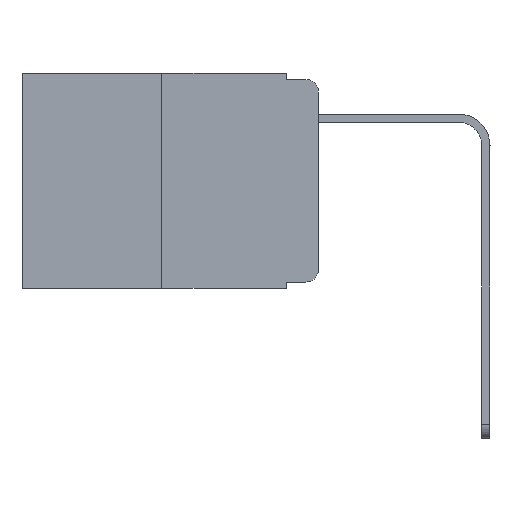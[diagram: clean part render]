
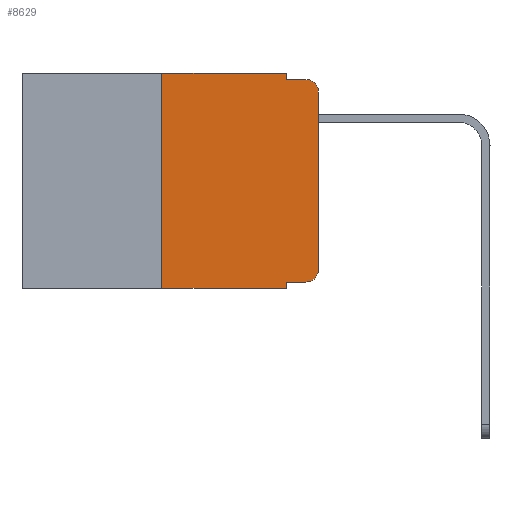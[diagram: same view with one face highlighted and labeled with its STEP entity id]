
A CAD part, left-side view. The second image highlights one B-rep face of the part: STEP entity #8629.
In plain terms, the highlighted planar face has unit normal (-1, 0, 0).
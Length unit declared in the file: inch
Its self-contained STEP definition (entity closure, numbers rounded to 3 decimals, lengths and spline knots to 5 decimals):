
#501 = VERTEX_POINT ( 'NONE', #15920 ) ;
#543 = VECTOR ( 'NONE', #5890, 39.37008 ) ;
#625 = AXIS2_PLACEMENT_3D ( 'NONE', #4485, #13887, #15265 ) ;
#633 = VERTEX_POINT ( 'NONE', #3951 ) ;
#739 = CARTESIAN_POINT ( 'NONE',  ( 0., 0.02, -0.01 ) ) ;
#911 = CARTESIAN_POINT ( 'NONE',  ( 0., 0., -0.03 ) ) ;
#965 = VERTEX_POINT ( 'NONE', #4037 ) ;
#992 = DIRECTION ( 'NONE',  ( 0., -1., 0. ) ) ;
#1010 = DIRECTION ( 'NONE',  ( -1., 0., 0. ) ) ;
#1401 = ORIENTED_EDGE ( 'NONE', *, *, #4761, .F. ) ;
#1824 = VECTOR ( 'NONE', #992, 39.37008 ) ;
#2135 = EDGE_CURVE ( 'NONE', #15957, #16170, #2227, .T. ) ;
#2227 = LINE ( 'NONE', #15925, #16977 ) ;
#2578 = DIRECTION ( 'NONE',  ( 0., 0., -1. ) ) ;
#2835 = DIRECTION ( 'NONE',  ( 0., -1., 0. ) ) ;
#3642 = DIRECTION ( 'NONE',  ( 0., 0., 1. ) ) ;
#3667 = VECTOR ( 'NONE', #15492, 39.37008 ) ;
#3936 = LINE ( 'NONE', #17284, #1824 ) ;
#3951 = CARTESIAN_POINT ( 'NONE',  ( 0., 0.02, -0.333 ) ) ;
#4037 = CARTESIAN_POINT ( 'NONE',  ( 0., 0.051, -0.333 ) ) ;
#4386 = VERTEX_POINT ( 'NONE', #13952 ) ;
#4485 = CARTESIAN_POINT ( 'NONE',  ( 0., 0.473, 0. ) ) ;
#4533 = FACE_OUTER_BOUND ( 'NONE', #6251, .T. ) ;
#4613 = DIRECTION ( 'NONE',  ( 0., 0., 1. ) ) ;
#4761 = EDGE_CURVE ( 'NONE', #4386, #15957, #12010, .T. ) ;
#5108 = LINE ( 'NONE', #12137, #16913 ) ;
#5312 = ORIENTED_EDGE ( 'NONE', *, *, #8524, .F. ) ;
#5323 = CARTESIAN_POINT ( 'NONE',  ( 0., 0.25, 0. ) ) ;
#5349 = ORIENTED_EDGE ( 'NONE', *, *, #17445, .T. ) ;
#5890 = DIRECTION ( 'NONE',  ( 0., 0., -1. ) ) ;
#5933 = VERTEX_POINT ( 'NONE', #739 ) ;
#6251 = EDGE_LOOP ( 'NONE', ( #5349, #10031, #16298, #17118, #11728, #1401, #11216, #5312, #8288, #10722 ) ) ;
#6370 = CARTESIAN_POINT ( 'NONE',  ( 0., 0.25, 0. ) ) ;
#6430 = CIRCLE ( 'NONE', #15039, 0.02 ) ;
#6477 = EDGE_CURVE ( 'NONE', #4386, #13748, #17028, .T. ) ;
#7370 = CARTESIAN_POINT ( 'NONE',  ( 0., 0.051, 0. ) ) ;
#7748 = CARTESIAN_POINT ( 'NONE',  ( 0., 0.02, -0.03 ) ) ;
#7802 = VECTOR ( 'NONE', #4613, 39.37008 ) ;
#8288 = ORIENTED_EDGE ( 'NONE', *, *, #13700, .T. ) ;
#8314 = EDGE_CURVE ( 'NONE', #633, #15771, #6430, .T. ) ;
#8524 = EDGE_CURVE ( 'NONE', #965, #13748, #15048, .T. ) ;
#8629 = ADVANCED_FACE ( 'NONE', ( #4533 ), #12532, .F. ) ;
#9054 = CARTESIAN_POINT ( 'NONE',  ( 0., 0.02, -0.313 ) ) ;
#9176 = DIRECTION ( 'NONE',  ( 0., -1., 0. ) ) ;
#9190 = EDGE_CURVE ( 'NONE', #16170, #501, #10177, .T. ) ;
#9458 = EDGE_CURVE ( 'NONE', #14039, #5933, #17158, .T. ) ;
#9473 = CARTESIAN_POINT ( 'NONE',  ( 0., 0.473, -0.343 ) ) ;
#9490 = DIRECTION ( 'NONE',  ( 0., -1., 0. ) ) ;
#10031 = ORIENTED_EDGE ( 'NONE', *, *, #9458, .T. ) ;
#10068 = CARTESIAN_POINT ( 'NONE',  ( 0., 0., 0. ) ) ;
#10177 = LINE ( 'NONE', #16508, #3667 ) ;
#10398 = DIRECTION ( 'NONE',  ( 0., 0., -1. ) ) ;
#10722 = ORIENTED_EDGE ( 'NONE', *, *, #8314, .T. ) ;
#11216 = ORIENTED_EDGE ( 'NONE', *, *, #6477, .T. ) ;
#11693 = EDGE_CURVE ( 'NONE', #501, #5933, #3936, .T. ) ;
#11728 = ORIENTED_EDGE ( 'NONE', *, *, #2135, .F. ) ;
#12010 = LINE ( 'NONE', #6370, #15853 ) ;
#12137 = CARTESIAN_POINT ( 'NONE',  ( 0., 0.051, -0.333 ) ) ;
#12532 = PLANE ( 'NONE',  #625 ) ;
#12641 = LINE ( 'NONE', #10068, #7802 ) ;
#13700 = EDGE_CURVE ( 'NONE', #965, #633, #5108, .T. ) ;
#13748 = VERTEX_POINT ( 'NONE', #15024 ) ;
#13764 = CARTESIAN_POINT ( 'NONE',  ( 0., 0.051, 0. ) ) ;
#13887 = DIRECTION ( 'NONE',  ( 1., 0., 0. ) ) ;
#13952 = CARTESIAN_POINT ( 'NONE',  ( 0., 0.25, -0.343 ) ) ;
#14039 = VERTEX_POINT ( 'NONE', #911 ) ;
#14680 = DIRECTION ( 'NONE',  ( -1., 0., 0. ) ) ;
#15024 = CARTESIAN_POINT ( 'NONE',  ( 0., 0.051, -0.343 ) ) ;
#15039 = AXIS2_PLACEMENT_3D ( 'NONE', #9054, #1010, #10398 ) ;
#15048 = LINE ( 'NONE', #13764, #543 ) ;
#15095 = AXIS2_PLACEMENT_3D ( 'NONE', #7748, #14680, #2578 ) ;
#15265 = DIRECTION ( 'NONE',  ( 0., 0., -1. ) ) ;
#15492 = DIRECTION ( 'NONE',  ( 0., 0., -1. ) ) ;
#15771 = VERTEX_POINT ( 'NONE', #17132 ) ;
#15853 = VECTOR ( 'NONE', #3642, 39.37008 ) ;
#15920 = CARTESIAN_POINT ( 'NONE',  ( 0., 0.051, -0.01 ) ) ;
#15925 = CARTESIAN_POINT ( 'NONE',  ( 0., 0.473, 0. ) ) ;
#15957 = VERTEX_POINT ( 'NONE', #5323 ) ;
#16170 = VERTEX_POINT ( 'NONE', #7370 ) ;
#16196 = VECTOR ( 'NONE', #2835, 39.37008 ) ;
#16298 = ORIENTED_EDGE ( 'NONE', *, *, #11693, .F. ) ;
#16508 = CARTESIAN_POINT ( 'NONE',  ( 0., 0.051, 0. ) ) ;
#16913 = VECTOR ( 'NONE', #9490, 39.37008 ) ;
#16977 = VECTOR ( 'NONE', #9176, 39.37008 ) ;
#17028 = LINE ( 'NONE', #9473, #16196 ) ;
#17118 = ORIENTED_EDGE ( 'NONE', *, *, #9190, .F. ) ;
#17132 = CARTESIAN_POINT ( 'NONE',  ( 0., 0., -0.313 ) ) ;
#17158 = CIRCLE ( 'NONE', #15095, 0.02 ) ;
#17284 = CARTESIAN_POINT ( 'NONE',  ( 0., 0.051, -0.01 ) ) ;
#17445 = EDGE_CURVE ( 'NONE', #15771, #14039, #12641, .T. ) ;
